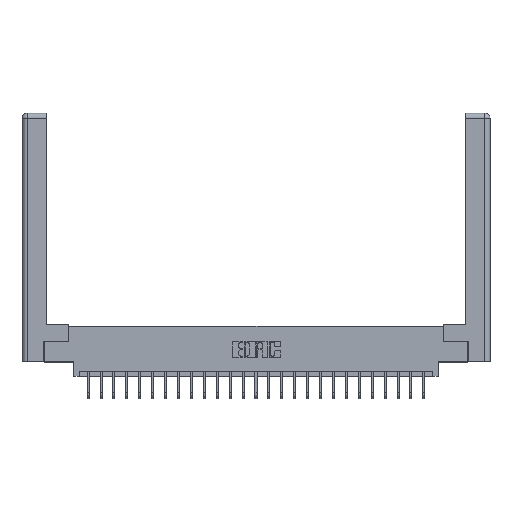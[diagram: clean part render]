
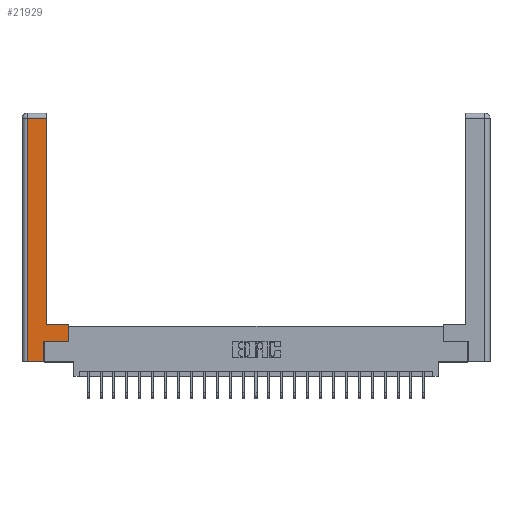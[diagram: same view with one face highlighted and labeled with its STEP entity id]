
A CAD part, top view. The second image highlights one B-rep face of the part: STEP entity #21929.
In plain terms, the highlighted planar face has unit normal (0, 0, 1).
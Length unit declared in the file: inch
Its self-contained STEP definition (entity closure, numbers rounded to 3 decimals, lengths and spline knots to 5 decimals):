
#274 = ORIENTED_EDGE ( 'NONE', *, *, #4744, .T. ) ;
#1027 = VERTEX_POINT ( 'NONE', #14835 ) ;
#1218 = CARTESIAN_POINT ( 'NONE',  ( 0.0615, 2.94, 0. ) ) ;
#1371 = DIRECTION ( 'NONE',  ( 0., 0., -1. ) ) ;
#1654 = CARTESIAN_POINT ( 'NONE',  ( 0.0615, 2.94, 0. ) ) ;
#1847 = CARTESIAN_POINT ( 'NONE',  ( 0.0615, 0., 0. ) ) ;
#2380 = VECTOR ( 'NONE', #11746, 39.37008 ) ;
#2989 = EDGE_LOOP ( 'NONE', ( #18488, #12202, #21635, #18061, #23705, #274, #7394, #19874 ) ) ;
#3160 = LINE ( 'NONE', #1218, #10642 ) ;
#3570 = EDGE_CURVE ( 'NONE', #7362, #11589, #20846, .T. ) ;
#4744 = EDGE_CURVE ( 'NONE', #11589, #12965, #18079, .T. ) ;
#4824 = DIRECTION ( 'NONE',  ( -1., 0., 0. ) ) ;
#5791 = VECTOR ( 'NONE', #13748, 39.37008 ) ;
#7093 = LINE ( 'NONE', #19465, #2380 ) ;
#7229 = CARTESIAN_POINT ( 'NONE',  ( 0.295, 2.94, 0. ) ) ;
#7362 = VERTEX_POINT ( 'NONE', #17235 ) ;
#7394 = ORIENTED_EDGE ( 'NONE', *, *, #9958, .T. ) ;
#8798 = VECTOR ( 'NONE', #24322, 39.37008 ) ;
#8977 = PLANE ( 'NONE',  #18102 ) ;
#9958 = EDGE_CURVE ( 'NONE', #12965, #14453, #19950, .T. ) ;
#10120 = CARTESIAN_POINT ( 'NONE',  ( 0.565, 0.45, 0. ) ) ;
#10642 = VECTOR ( 'NONE', #4824, 39.37008 ) ;
#11589 = VERTEX_POINT ( 'NONE', #11894 ) ;
#11746 = DIRECTION ( 'NONE',  ( -1., 0., 0. ) ) ;
#11894 = CARTESIAN_POINT ( 'NONE',  ( 0.265, 0.245, 0. ) ) ;
#12087 = LINE ( 'NONE', #15769, #5791 ) ;
#12202 = ORIENTED_EDGE ( 'NONE', *, *, #20073, .T. ) ;
#12850 = CARTESIAN_POINT ( 'NONE',  ( 0., 0., 0. ) ) ;
#12965 = VERTEX_POINT ( 'NONE', #20487 ) ;
#13389 = VERTEX_POINT ( 'NONE', #1847 ) ;
#13641 = DIRECTION ( 'NONE',  ( 1., 0., 0. ) ) ;
#13748 = DIRECTION ( 'NONE',  ( 0., 1., 0. ) ) ;
#14453 = VERTEX_POINT ( 'NONE', #10120 ) ;
#14625 = DIRECTION ( 'NONE',  ( 0., 1., 0. ) ) ;
#14826 = CARTESIAN_POINT ( 'NONE',  ( 0.565, 0.245, 0. ) ) ;
#14835 = CARTESIAN_POINT ( 'NONE',  ( 0.295, 0.45, 0. ) ) ;
#15256 = VECTOR ( 'NONE', #23229, 39.37008 ) ;
#15769 = CARTESIAN_POINT ( 'NONE',  ( 0.295, 3., 0. ) ) ;
#17235 = CARTESIAN_POINT ( 'NONE',  ( 0.265, 0., 0. ) ) ;
#17338 = EDGE_CURVE ( 'NONE', #14453, #1027, #7093, .T. ) ;
#18061 = ORIENTED_EDGE ( 'NONE', *, *, #18710, .T. ) ;
#18079 = LINE ( 'NONE', #14826, #19854 ) ;
#18102 = AXIS2_PLACEMENT_3D ( 'NONE', #12850, #1371, #22656 ) ;
#18488 = ORIENTED_EDGE ( 'NONE', *, *, #22790, .T. ) ;
#18548 = CARTESIAN_POINT ( 'NONE',  ( 0.265, 0.245, 0. ) ) ;
#18710 = EDGE_CURVE ( 'NONE', #13389, #7362, #19752, .T. ) ;
#18992 = VECTOR ( 'NONE', #23872, 39.37008 ) ;
#19465 = CARTESIAN_POINT ( 'NONE',  ( 0.295, 0.45, 0. ) ) ;
#19752 = LINE ( 'NONE', #21223, #15256 ) ;
#19854 = VECTOR ( 'NONE', #13641, 39.37008 ) ;
#19874 = ORIENTED_EDGE ( 'NONE', *, *, #17338, .T. ) ;
#19950 = LINE ( 'NONE', #22606, #21775 ) ;
#20073 = EDGE_CURVE ( 'NONE', #21848, #23903, #3160, .T. ) ;
#20487 = CARTESIAN_POINT ( 'NONE',  ( 0.565, 0.245, 0. ) ) ;
#20846 = LINE ( 'NONE', #18548, #8798 ) ;
#21223 = CARTESIAN_POINT ( 'NONE',  ( 0.265, 0., 0. ) ) ;
#21480 = FACE_OUTER_BOUND ( 'NONE', #2989, .T. ) ;
#21635 = ORIENTED_EDGE ( 'NONE', *, *, #23682, .T. ) ;
#21775 = VECTOR ( 'NONE', #14625, 39.37008 ) ;
#21848 = VERTEX_POINT ( 'NONE', #7229 ) ;
#21929 = ADVANCED_FACE ( 'NONE', ( #21480 ), #8977, .F. ) ;
#22038 = CARTESIAN_POINT ( 'NONE',  ( 0.0615, 0., 0. ) ) ;
#22606 = CARTESIAN_POINT ( 'NONE',  ( 0.565, 0.45, 0. ) ) ;
#22656 = DIRECTION ( 'NONE',  ( -1., 0., 0. ) ) ;
#22790 = EDGE_CURVE ( 'NONE', #1027, #21848, #12087, .T. ) ;
#23229 = DIRECTION ( 'NONE',  ( 1., 0., 0. ) ) ;
#23682 = EDGE_CURVE ( 'NONE', #23903, #13389, #24085, .T. ) ;
#23705 = ORIENTED_EDGE ( 'NONE', *, *, #3570, .T. ) ;
#23872 = DIRECTION ( 'NONE',  ( 0., -1., 0. ) ) ;
#23903 = VERTEX_POINT ( 'NONE', #1654 ) ;
#24085 = LINE ( 'NONE', #22038, #18992 ) ;
#24322 = DIRECTION ( 'NONE',  ( 0., 1., 0. ) ) ;
